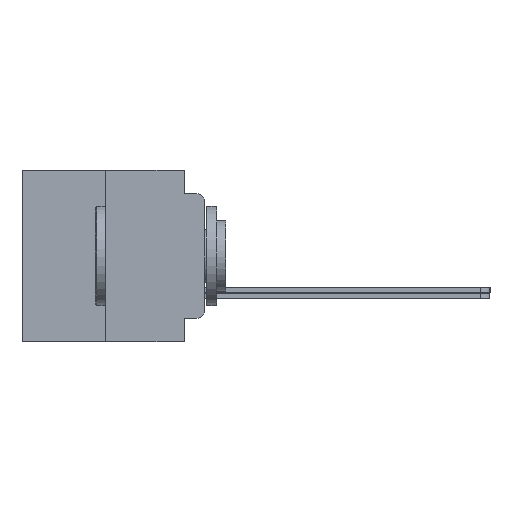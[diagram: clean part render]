
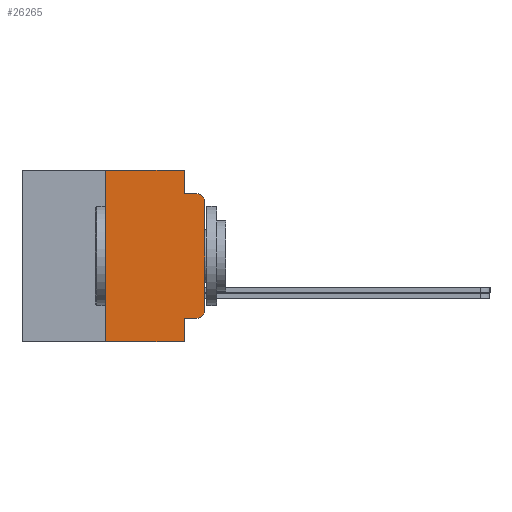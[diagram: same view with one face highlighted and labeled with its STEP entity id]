
A CAD part, left-side view. The second image highlights one B-rep face of the part: STEP entity #26265.
In plain terms, the highlighted planar face has unit normal (-1, 0, 0).
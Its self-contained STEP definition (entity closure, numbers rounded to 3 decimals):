
#65 = ORIENTED_EDGE ( 'NONE', *, *, #6253, .F. ) ;
#146 = CARTESIAN_POINT ( 'NONE',  ( -75.603, 6.35, -5.486 ) ) ;
#394 = CARTESIAN_POINT ( 'NONE',  ( -75.603, 0.508, 3.467 ) ) ;
#1019 = EDGE_CURVE ( 'NONE', #19596, #3034, #26612, .T. ) ;
#1079 = VECTOR ( 'NONE', #9451, 1000. ) ;
#1128 = ORIENTED_EDGE ( 'NONE', *, *, #5828, .T. ) ;
#2315 = ORIENTED_EDGE ( 'NONE', *, *, #27498, .F. ) ;
#2623 = VECTOR ( 'NONE', #28345, 1000. ) ;
#2847 = EDGE_CURVE ( 'NONE', #10733, #24255, #10905, .T. ) ;
#2934 = CARTESIAN_POINT ( 'NONE',  ( -75.603, 0.508, -3.467 ) ) ;
#3034 = VERTEX_POINT ( 'NONE', #24466 ) ;
#3295 = FACE_OUTER_BOUND ( 'NONE', #7109, .T. ) ;
#4172 = VERTEX_POINT ( 'NONE', #12072 ) ;
#4181 = DIRECTION ( 'NONE',  ( 0., 0., 1. ) ) ;
#4282 = LINE ( 'NONE', #15448, #18493 ) ;
#4420 = DIRECTION ( 'NONE',  ( 0., 0., -1. ) ) ;
#5723 = VECTOR ( 'NONE', #15419, 1000. ) ;
#5751 = VERTEX_POINT ( 'NONE', #6745 ) ;
#5828 = EDGE_CURVE ( 'NONE', #3034, #26456, #7634, .T. ) ;
#6001 = VECTOR ( 'NONE', #4181, 1000. ) ;
#6131 = DIRECTION ( 'NONE',  ( 0., -1., 0. ) ) ;
#6253 = EDGE_CURVE ( 'NONE', #24255, #17883, #21106, .T. ) ;
#6745 = CARTESIAN_POINT ( 'NONE',  ( -75.603, 6.35, -5.486 ) ) ;
#7027 = DIRECTION ( 'NONE',  ( 1., 0., 0. ) ) ;
#7109 = EDGE_LOOP ( 'NONE', ( #20805, #11941, #1128, #19279, #65, #7968, #12164, #2315, #27888, #11411 ) ) ;
#7374 = VERTEX_POINT ( 'NONE', #14207 ) ;
#7634 = LINE ( 'NONE', #27231, #1079 ) ;
#7763 = DIRECTION ( 'NONE',  ( 0., -1., 0. ) ) ;
#7797 = DIRECTION ( 'NONE',  ( -1., 0., 0. ) ) ;
#7848 = CARTESIAN_POINT ( 'NONE',  ( -75.603, 1.295, -3.975 ) ) ;
#7968 = ORIENTED_EDGE ( 'NONE', *, *, #2847, .F. ) ;
#8343 = VECTOR ( 'NONE', #26347, 1000. ) ;
#8704 = EDGE_CURVE ( 'NONE', #4172, #10733, #8834, .T. ) ;
#8834 = LINE ( 'NONE', #26291, #2623 ) ;
#9370 = DIRECTION ( 'NONE',  ( 0., 0., -1. ) ) ;
#9451 = DIRECTION ( 'NONE',  ( 0., 0., 1. ) ) ;
#10733 = VERTEX_POINT ( 'NONE', #20196 ) ;
#10905 = LINE ( 'NONE', #26132, #5723 ) ;
#11095 = PLANE ( 'NONE',  #18652 ) ;
#11411 = ORIENTED_EDGE ( 'NONE', *, *, #12912, .F. ) ;
#11769 = CARTESIAN_POINT ( 'NONE',  ( -75.603, 0., 3.467 ) ) ;
#11941 = ORIENTED_EDGE ( 'NONE', *, *, #1019, .T. ) ;
#12072 = CARTESIAN_POINT ( 'NONE',  ( -75.603, 6.35, 5.486 ) ) ;
#12164 = ORIENTED_EDGE ( 'NONE', *, *, #8704, .F. ) ;
#12265 = DIRECTION ( 'NONE',  ( 0., 0., -1. ) ) ;
#12912 = EDGE_CURVE ( 'NONE', #27213, #7374, #26011, .T. ) ;
#14206 = AXIS2_PLACEMENT_3D ( 'NONE', #394, #20268, #9370 ) ;
#14207 = CARTESIAN_POINT ( 'NONE',  ( -75.603, 1.295, -5.486 ) ) ;
#15256 = VECTOR ( 'NONE', #6131, 1000. ) ;
#15419 = DIRECTION ( 'NONE',  ( 0., 0., -1. ) ) ;
#15446 = CARTESIAN_POINT ( 'NONE',  ( -75.603, 1.295, 0. ) ) ;
#15448 = CARTESIAN_POINT ( 'NONE',  ( -75.603, 11.684, -5.486 ) ) ;
#16951 = AXIS2_PLACEMENT_3D ( 'NONE', #2934, #7797, #12265 ) ;
#17066 = EDGE_CURVE ( 'NONE', #26456, #17883, #22634, .T. ) ;
#17593 = EDGE_CURVE ( 'NONE', #5751, #7374, #4282, .T. ) ;
#17883 = VERTEX_POINT ( 'NONE', #27416 ) ;
#18463 = LINE ( 'NONE', #146, #6001 ) ;
#18493 = VECTOR ( 'NONE', #23919, 1000. ) ;
#18652 = AXIS2_PLACEMENT_3D ( 'NONE', #19978, #7027, #4420 ) ;
#19214 = CARTESIAN_POINT ( 'NONE',  ( -75.603, 0.508, -3.975 ) ) ;
#19279 = ORIENTED_EDGE ( 'NONE', *, *, #17066, .T. ) ;
#19596 = VERTEX_POINT ( 'NONE', #19214 ) ;
#19978 = CARTESIAN_POINT ( 'NONE',  ( -75.603, 11.684, 5.486 ) ) ;
#20196 = CARTESIAN_POINT ( 'NONE',  ( -75.603, 1.295, 5.486 ) ) ;
#20268 = DIRECTION ( 'NONE',  ( -1., 0., 0. ) ) ;
#20805 = ORIENTED_EDGE ( 'NONE', *, *, #25400, .T. ) ;
#21106 = LINE ( 'NONE', #24088, #15256 ) ;
#21312 = LINE ( 'NONE', #7848, #25509 ) ;
#22634 = CIRCLE ( 'NONE', #14206, 0.508 ) ;
#22923 = CARTESIAN_POINT ( 'NONE',  ( -75.603, 1.295, -3.975 ) ) ;
#23919 = DIRECTION ( 'NONE',  ( 0., -1., 0. ) ) ;
#24088 = CARTESIAN_POINT ( 'NONE',  ( -75.603, 1.295, 3.975 ) ) ;
#24255 = VERTEX_POINT ( 'NONE', #24648 ) ;
#24466 = CARTESIAN_POINT ( 'NONE',  ( -75.603, 0., -3.467 ) ) ;
#24648 = CARTESIAN_POINT ( 'NONE',  ( -75.603, 1.295, 3.975 ) ) ;
#25400 = EDGE_CURVE ( 'NONE', #27213, #19596, #21312, .T. ) ;
#25509 = VECTOR ( 'NONE', #7763, 1000. ) ;
#26011 = LINE ( 'NONE', #15446, #8343 ) ;
#26132 = CARTESIAN_POINT ( 'NONE',  ( -75.603, 1.295, 0. ) ) ;
#26265 = ADVANCED_FACE ( 'NONE', ( #3295 ), #11095, .F. ) ;
#26291 = CARTESIAN_POINT ( 'NONE',  ( -75.603, 11.684, 5.486 ) ) ;
#26347 = DIRECTION ( 'NONE',  ( 0., 0., -1. ) ) ;
#26456 = VERTEX_POINT ( 'NONE', #11769 ) ;
#26612 = CIRCLE ( 'NONE', #16951, 0.508 ) ;
#27213 = VERTEX_POINT ( 'NONE', #22923 ) ;
#27231 = CARTESIAN_POINT ( 'NONE',  ( -75.603, 0., 5.486 ) ) ;
#27416 = CARTESIAN_POINT ( 'NONE',  ( -75.603, 0.508, 3.975 ) ) ;
#27498 = EDGE_CURVE ( 'NONE', #5751, #4172, #18463, .T. ) ;
#27888 = ORIENTED_EDGE ( 'NONE', *, *, #17593, .T. ) ;
#28345 = DIRECTION ( 'NONE',  ( 0., -1., 0. ) ) ;
